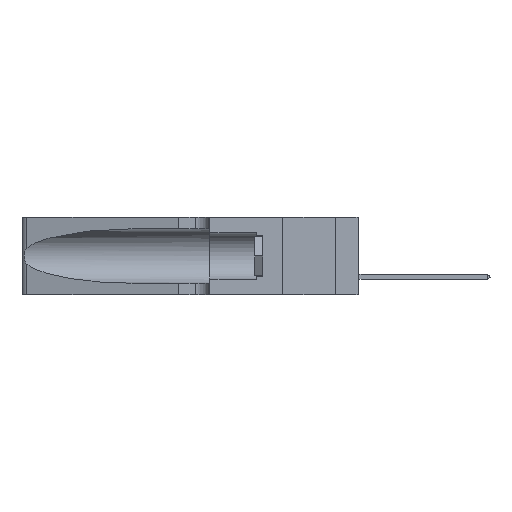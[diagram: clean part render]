
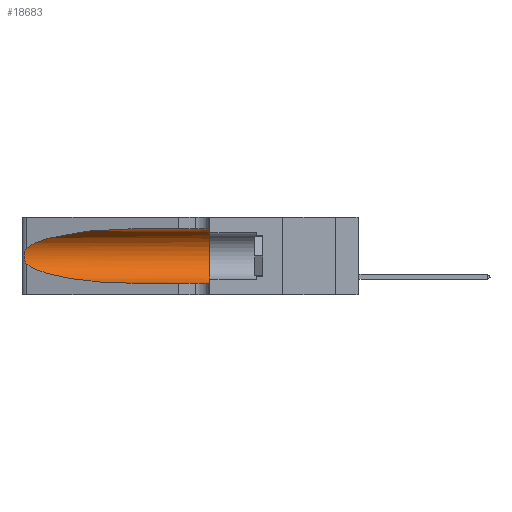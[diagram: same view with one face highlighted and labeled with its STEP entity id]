
A CAD part, left-side view. The second image highlights one B-rep face of the part: STEP entity #18683.
In plain terms, the highlighted cylindrical face has radius 3.308 mm (diameter 6.617 mm), a partial arc.
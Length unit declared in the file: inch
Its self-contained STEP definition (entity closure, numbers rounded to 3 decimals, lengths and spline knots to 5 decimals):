
#178 = VERTEX_POINT ( 'NONE', #26330 ) ;
#1216 = CARTESIAN_POINT ( 'NONE',  ( 0.1305, 1.61858, 0.05475 ) ) ;
#1450 = CARTESIAN_POINT ( 'NONE',  ( 0.1305, 1.61858, 0.31525 ) ) ;
#1523 = CARTESIAN_POINT ( 'NONE',  ( 0.26017, 1.23833, 0.17102 ) ) ;
#1555 = CARTESIAN_POINT ( 'NONE',  ( 0.18966, 0.96281, 0.05475 ) ) ;
#1689 = CARTESIAN_POINT ( 'NONE',  ( 0.25555, 1.22993, 0.14849 ) ) ;
#2203 = VERTEX_POINT ( 'NONE', #10036 ) ;
#2230 = ORIENTED_EDGE ( 'NONE', *, *, #39352, .T. ) ;
#3284 = CYLINDRICAL_SURFACE ( 'NONE', #21586, 0.13025 ) ;
#3855 = CARTESIAN_POINT ( 'NONE',  ( 0.1305, 0.72297, 0.31525 ) ) ;
#4625 = EDGE_CURVE ( 'NONE', #2203, #20775, #45941, .T. ) ;
#4688 = DIRECTION ( 'NONE',  ( 0., 0., -1. ) ) ;
#5035 = EDGE_LOOP ( 'NONE', ( #2230, #46668, #26106, #46940, #26037, #24291 ) ) ;
#5456 = CARTESIAN_POINT ( 'NONE',  ( 0.25639, 1.23186, 0.15144 ) ) ;
#5609 = CARTESIAN_POINT ( 'NONE',  ( 0.25789, 1.23486, 0.15765 ) ) ;
#9810 = CARTESIAN_POINT ( 'NONE',  ( 0.26075, 1.23896, 0.178 ) ) ;
#9988 = CARTESIAN_POINT ( 'NONE',  ( 0.25856, 1.23593, 0.16098 ) ) ;
#10036 = CARTESIAN_POINT ( 'NONE',  ( 0.25487, 1.22718, 0.14631 ) ) ;
#12195 = VERTEX_POINT ( 'NONE', #49626 ) ;
#12853 = CARTESIAN_POINT ( 'NONE',  ( 0.25487, 1.22718, 0.22369 ) ) ;
#13197 = DIRECTION ( 'NONE',  ( 0., -1., 0. ) ) ;
#15759 = CARTESIAN_POINT ( 'NONE',  ( 0.18966, 0.96281, 0.31525 ) ) ;
#16083 = DIRECTION ( 'NONE',  ( 0., 1., 0. ) ) ;
#16439 = CARTESIAN_POINT ( 'NONE',  ( 0.2373, 1.15595, 0.28018 ) ) ;
#16512 = VECTOR ( 'NONE', #13197, 39.37008 ) ;
#17015 = CARTESIAN_POINT ( 'NONE',  ( 0.25854, 1.2359, 0.20912 ) ) ;
#18048 = CARTESIAN_POINT ( 'NONE',  ( 0.1305, 0.35, 0.05475 ) ) ;
#18683 = ADVANCED_FACE ( 'NONE', ( #31360 ), #3284, .F. ) ;
#20775 = VERTEX_POINT ( 'NONE', #45049 ) ;
#20805 = EDGE_CURVE ( 'NONE', #12195, #2203, #22416, .T. ) ;
#21476 =( BOUNDED_CURVE ( )  B_SPLINE_CURVE ( 3, ( #3855, #15759, #16439, #12853 ),
 .UNSPECIFIED., .F., .F. ) 
 B_SPLINE_CURVE_WITH_KNOTS ( ( 4, 4 ),
 ( 1.5708, 2.84003 ),
 .UNSPECIFIED. ) 
 CURVE ( )  GEOMETRIC_REPRESENTATION_ITEM ( )  RATIONAL_B_SPLINE_CURVE ( ( 1., 0.87, 0.87, 1. ) ) 
 REPRESENTATION_ITEM ( '' )  );
#21586 = AXIS2_PLACEMENT_3D ( 'NONE', #43795, #40168, #4688 ) ;
#22416 = B_SPLINE_CURVE_WITH_KNOTS ( 'NONE', 3,
 ( #48453, #32895, #44875, #25054, #17015, #48799, #36637, #9810, #1523, #9988, #5609, #5456, #1689, #37155 ),
 .UNSPECIFIED., .F., .F.,
 ( 4, 2, 2, 2, 2, 2, 4 ),
 ( 0., 0.00027, 0.00053, 0.00107, 0.0016, 0.00187, 0.00214 ),
 .UNSPECIFIED. ) ;
#24264 = VERTEX_POINT ( 'NONE', #18048 ) ;
#24291 = ORIENTED_EDGE ( 'NONE', *, *, #38636, .F. ) ;
#25054 = CARTESIAN_POINT ( 'NONE',  ( 0.25787, 1.23484, 0.2124 ) ) ;
#26037 = ORIENTED_EDGE ( 'NONE', *, *, #34116, .F. ) ;
#26106 = ORIENTED_EDGE ( 'NONE', *, *, #4625, .T. ) ;
#26330 = CARTESIAN_POINT ( 'NONE',  ( 0.1305, 0.72297, 0.31525 ) ) ;
#28580 = VECTOR ( 'NONE', #32910, 39.37008 ) ;
#31360 = FACE_OUTER_BOUND ( 'NONE', #5035, .T. ) ;
#31632 = CARTESIAN_POINT ( 'NONE',  ( 0.1305, 0.35, 0.185 ) ) ;
#32895 = CARTESIAN_POINT ( 'NONE',  ( 0.25555, 1.22994, 0.2215 ) ) ;
#32910 = DIRECTION ( 'NONE',  ( 0., -1., 0. ) ) ;
#33669 = EDGE_CURVE ( 'NONE', #20775, #24264, #50623, .T. ) ;
#34116 = EDGE_CURVE ( 'NONE', #45505, #24264, #37041, .T. ) ;
#35537 = DIRECTION ( 'NONE',  ( 0., 0., 1. ) ) ;
#35628 = AXIS2_PLACEMENT_3D ( 'NONE', #31632, #16083, #35537 ) ;
#36056 = LINE ( 'NONE', #1450, #16512 ) ;
#36512 = CARTESIAN_POINT ( 'NONE',  ( 0.25487, 1.22718, 0.14631 ) ) ;
#36637 = CARTESIAN_POINT ( 'NONE',  ( 0.26075, 1.23896, 0.19203 ) ) ;
#37041 = CIRCLE ( 'NONE', #35628, 0.13025 ) ;
#37155 = CARTESIAN_POINT ( 'NONE',  ( 0.25487, 1.22718, 0.14631 ) ) ;
#38599 = CARTESIAN_POINT ( 'NONE',  ( 0.1305, 0.35, 0.31525 ) ) ;
#38636 = EDGE_CURVE ( 'NONE', #178, #45505, #36056, .T. ) ;
#39352 = EDGE_CURVE ( 'NONE', #178, #12195, #21476, .T. ) ;
#40168 = DIRECTION ( 'NONE',  ( 0., -1., 0. ) ) ;
#43795 = CARTESIAN_POINT ( 'NONE',  ( 0.1305, 1.61858, 0.185 ) ) ;
#44591 = CARTESIAN_POINT ( 'NONE',  ( 0.1305, 0.72297, 0.05475 ) ) ;
#44875 = CARTESIAN_POINT ( 'NONE',  ( 0.25639, 1.23184, 0.21858 ) ) ;
#45049 = CARTESIAN_POINT ( 'NONE',  ( 0.1305, 0.72297, 0.05475 ) ) ;
#45505 = VERTEX_POINT ( 'NONE', #38599 ) ;
#45941 =( BOUNDED_CURVE ( )  B_SPLINE_CURVE ( 3, ( #36512, #48340, #1555, #44591 ),
 .UNSPECIFIED., .F., .F. ) 
 B_SPLINE_CURVE_WITH_KNOTS ( ( 4, 4 ),
 ( 3.44316, 4.71239 ),
 .UNSPECIFIED. ) 
 CURVE ( )  GEOMETRIC_REPRESENTATION_ITEM ( )  RATIONAL_B_SPLINE_CURVE ( ( 1., 0.87, 0.87, 1. ) ) 
 REPRESENTATION_ITEM ( '' )  );
#46668 = ORIENTED_EDGE ( 'NONE', *, *, #20805, .T. ) ;
#46940 = ORIENTED_EDGE ( 'NONE', *, *, #33669, .T. ) ;
#48340 = CARTESIAN_POINT ( 'NONE',  ( 0.2373, 1.15595, 0.08982 ) ) ;
#48453 = CARTESIAN_POINT ( 'NONE',  ( 0.25487, 1.22718, 0.22369 ) ) ;
#48799 = CARTESIAN_POINT ( 'NONE',  ( 0.26018, 1.23835, 0.19895 ) ) ;
#49626 = CARTESIAN_POINT ( 'NONE',  ( 0.25487, 1.22718, 0.22369 ) ) ;
#50623 = LINE ( 'NONE', #1216, #28580 ) ;
